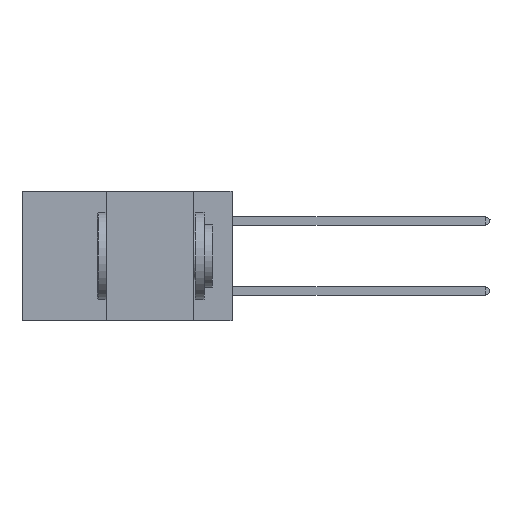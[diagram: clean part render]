
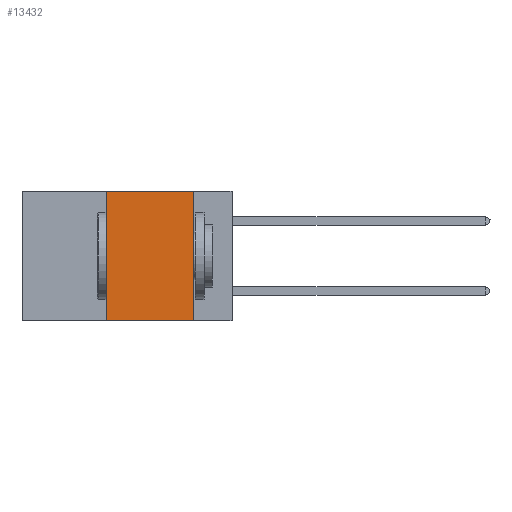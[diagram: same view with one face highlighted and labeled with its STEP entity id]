
A CAD part, left-side view. The second image highlights one B-rep face of the part: STEP entity #13432.
In plain terms, the highlighted planar face has unit normal (-1, 0, 0).
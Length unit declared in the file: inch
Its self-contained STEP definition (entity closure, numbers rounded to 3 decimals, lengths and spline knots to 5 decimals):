
#330 = CARTESIAN_POINT ( 'NONE',  ( 0., 0.36, -0.37 ) ) ;
#375 = DIRECTION ( 'NONE',  ( 0., -1., 0. ) ) ;
#472 = EDGE_CURVE ( 'NONE', #13163, #13613, #8552, .T. ) ;
#871 = DIRECTION ( 'NONE',  ( 0., 0., -1. ) ) ;
#1065 = VERTEX_POINT ( 'NONE', #12226 ) ;
#1153 = CARTESIAN_POINT ( 'NONE',  ( 0., 0.6, 0. ) ) ;
#1256 = CARTESIAN_POINT ( 'NONE',  ( 0., 0.11, 0. ) ) ;
#1681 = CARTESIAN_POINT ( 'NONE',  ( 0., 0.6, -0.37 ) ) ;
#1772 = ORIENTED_EDGE ( 'NONE', *, *, #13689, .T. ) ;
#2312 = ORIENTED_EDGE ( 'NONE', *, *, #7570, .F. ) ;
#2381 = PLANE ( 'NONE',  #14698 ) ;
#2506 = DIRECTION ( 'NONE',  ( 0., 0., 1. ) ) ;
#2744 = CARTESIAN_POINT ( 'NONE',  ( 0., 0.36, 0. ) ) ;
#3368 = CARTESIAN_POINT ( 'NONE',  ( 0., 0.11, -0.37 ) ) ;
#3623 = LINE ( 'NONE', #1153, #12785 ) ;
#4501 = ORIENTED_EDGE ( 'NONE', *, *, #472, .F. ) ;
#5743 = VECTOR ( 'NONE', #871, 39.37008 ) ;
#5985 = DIRECTION ( 'NONE',  ( 1., 0., 0. ) ) ;
#6048 = DIRECTION ( 'NONE',  ( 0., -1., 0. ) ) ;
#6191 = EDGE_CURVE ( 'NONE', #1065, #8598, #8931, .T. ) ;
#7570 = EDGE_CURVE ( 'NONE', #13613, #1065, #3623, .T. ) ;
#7807 = VECTOR ( 'NONE', #2506, 39.37008 ) ;
#8145 = CARTESIAN_POINT ( 'NONE',  ( 0., 0.6, 0. ) ) ;
#8438 = CARTESIAN_POINT ( 'NONE',  ( 0., 0.36, 0. ) ) ;
#8552 = LINE ( 'NONE', #8438, #7807 ) ;
#8598 = VERTEX_POINT ( 'NONE', #3368 ) ;
#8931 = LINE ( 'NONE', #1256, #5743 ) ;
#9048 = EDGE_LOOP ( 'NONE', ( #12106, #2312, #4501, #1772 ) ) ;
#10231 = FACE_OUTER_BOUND ( 'NONE', #9048, .T. ) ;
#12106 = ORIENTED_EDGE ( 'NONE', *, *, #6191, .F. ) ;
#12226 = CARTESIAN_POINT ( 'NONE',  ( 0., 0.11, 0. ) ) ;
#12785 = VECTOR ( 'NONE', #6048, 39.37008 ) ;
#12831 = VECTOR ( 'NONE', #375, 39.37008 ) ;
#13163 = VERTEX_POINT ( 'NONE', #330 ) ;
#13191 = LINE ( 'NONE', #1681, #12831 ) ;
#13432 = ADVANCED_FACE ( 'NONE', ( #10231 ), #2381, .F. ) ;
#13613 = VERTEX_POINT ( 'NONE', #2744 ) ;
#13689 = EDGE_CURVE ( 'NONE', #13163, #8598, #13191, .T. ) ;
#14318 = DIRECTION ( 'NONE',  ( 0., 0., -1. ) ) ;
#14698 = AXIS2_PLACEMENT_3D ( 'NONE', #8145, #5985, #14318 ) ;
